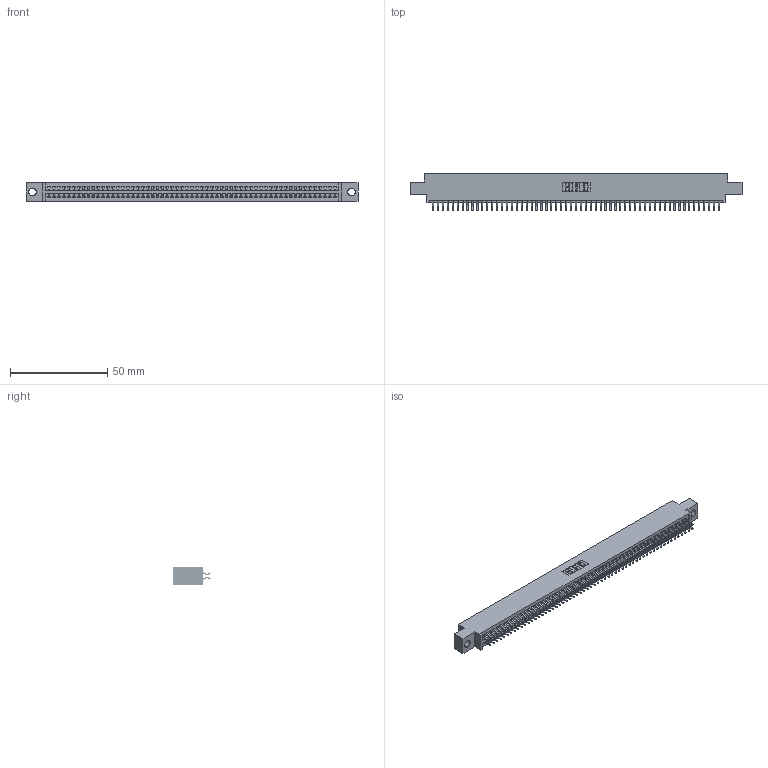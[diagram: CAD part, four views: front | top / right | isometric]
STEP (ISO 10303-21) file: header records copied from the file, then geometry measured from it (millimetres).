
FILE_DESCRIPTION (( 'STEP AP203' ), '1' );
FILE_NAME ('395-118-556-804.STEP', '2021-06-17T20:21:33', ( '' ), ( '' ), 'SwSTEP 2.0', 'SolidWorks 2020', '' );
FILE_SCHEMA (( 'CONFIG_CONTROL_DESIGN' ));
Length unit declared in the file: inch
Products named in the file (3): 345-292-001_556 Tail; 395-118-556-804; 345 Part_0.170 Offset - 0.156 Dia-TI
Assembly tree (119 placements, depth 2):
  395-118-556-804
    345 Part_0.170 Offset - 0.156 Dia-TI
    345-292-001_556 Tail  x118
Bounding box: 171.07 x 19.24 x 9.4 mm (x, y, z)
Volume: 16551.6 mm3; surface area: 24687.1 mm2
Topology: 119 solids, 119 shells, 6752 faces, 20095 edges, 13238 vertices
Faces by surface type: plane 4464, cylinder 2288
Entity records: 44775 total; most frequent: CARTESIAN_POINT 7510, ORIENTED_EDGE 7430, DIRECTION 6587, EDGE_CURVE 3715, VECTOR 3339, LINE 3339, VERTEX_POINT 2474, AXIS2_PLACEMENT_3D 1624
